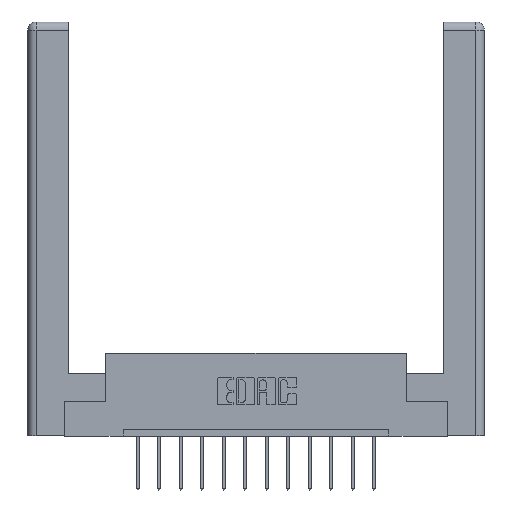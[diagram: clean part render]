
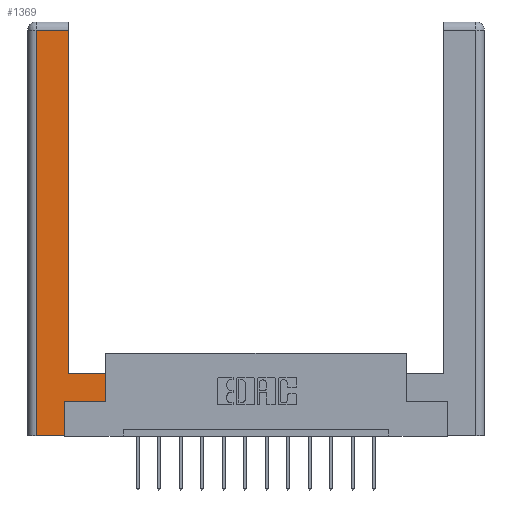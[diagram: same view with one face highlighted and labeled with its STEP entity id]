
A CAD part, top view. The second image highlights one B-rep face of the part: STEP entity #1369.
In plain terms, the highlighted planar face has unit normal (0, 0, 1).
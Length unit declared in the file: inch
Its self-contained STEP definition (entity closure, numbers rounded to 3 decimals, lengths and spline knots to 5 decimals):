
#84 = EDGE_CURVE ( 'NONE', #9626, #12899, #12550, .T. ) ;
#454 = EDGE_CURVE ( 'NONE', #13436, #5802, #12744, .T. ) ;
#967 = CARTESIAN_POINT ( 'NONE',  ( 0.565, 0.245, 0. ) ) ;
#1030 = ORIENTED_EDGE ( 'NONE', *, *, #15448, .T. ) ;
#1088 = CARTESIAN_POINT ( 'NONE',  ( 0.0615, 0., 0. ) ) ;
#1291 = VERTEX_POINT ( 'NONE', #6647 ) ;
#1369 = ADVANCED_FACE ( 'NONE', ( #5963 ), #9973, .F. ) ;
#1589 = LINE ( 'NONE', #15009, #4022 ) ;
#1873 = CARTESIAN_POINT ( 'NONE',  ( 0.265, 0.245, 0. ) ) ;
#1996 = EDGE_CURVE ( 'NONE', #12899, #4036, #5397, .T. ) ;
#2289 = CARTESIAN_POINT ( 'NONE',  ( 0.0615, 2.94, 0. ) ) ;
#2764 = EDGE_CURVE ( 'NONE', #1291, #13004, #11936, .T. ) ;
#2910 = LINE ( 'NONE', #1873, #14109 ) ;
#3070 = ORIENTED_EDGE ( 'NONE', *, *, #1996, .T. ) ;
#3510 = EDGE_LOOP ( 'NONE', ( #1030, #5829, #11685, #3070, #14769, #4694, #4431, #4227 ) ) ;
#3810 = DIRECTION ( 'NONE',  ( 0., 1., 0. ) ) ;
#4022 = VECTOR ( 'NONE', #10203, 39.37008 ) ;
#4036 = VERTEX_POINT ( 'NONE', #5295 ) ;
#4135 = DIRECTION ( 'NONE',  ( 0., 0., -1. ) ) ;
#4186 = CARTESIAN_POINT ( 'NONE',  ( 0., 0., 0. ) ) ;
#4227 = ORIENTED_EDGE ( 'NONE', *, *, #454, .T. ) ;
#4431 = ORIENTED_EDGE ( 'NONE', *, *, #12311, .T. ) ;
#4521 = VECTOR ( 'NONE', #15056, 39.37008 ) ;
#4586 = DIRECTION ( 'NONE',  ( -1., 0., 0. ) ) ;
#4694 = ORIENTED_EDGE ( 'NONE', *, *, #2764, .T. ) ;
#4949 = EDGE_CURVE ( 'NONE', #9069, #9626, #10179, .T. ) ;
#5267 = DIRECTION ( 'NONE',  ( -1., 0., 0. ) ) ;
#5295 = CARTESIAN_POINT ( 'NONE',  ( 0.265, 0., 0. ) ) ;
#5397 = LINE ( 'NONE', #14403, #10457 ) ;
#5498 = CARTESIAN_POINT ( 'NONE',  ( 0.295, 0.45, 0. ) ) ;
#5618 = DIRECTION ( 'NONE',  ( 0., 1., 0. ) ) ;
#5802 = VERTEX_POINT ( 'NONE', #6355 ) ;
#5829 = ORIENTED_EDGE ( 'NONE', *, *, #4949, .T. ) ;
#5963 = FACE_OUTER_BOUND ( 'NONE', #3510, .T. ) ;
#6355 = CARTESIAN_POINT ( 'NONE',  ( 0.295, 0.45, 0. ) ) ;
#6647 = CARTESIAN_POINT ( 'NONE',  ( 0.265, 0.245, 0. ) ) ;
#6973 = DIRECTION ( 'NONE',  ( 1., 0., 0. ) ) ;
#8461 = CARTESIAN_POINT ( 'NONE',  ( 0.295, 2.94, 0. ) ) ;
#8930 = CARTESIAN_POINT ( 'NONE',  ( 0.0615, 0., 0. ) ) ;
#8996 = VECTOR ( 'NONE', #11958, 39.37008 ) ;
#9069 = VERTEX_POINT ( 'NONE', #8461 ) ;
#9594 = VECTOR ( 'NONE', #3810, 39.37008 ) ;
#9626 = VERTEX_POINT ( 'NONE', #14780 ) ;
#9973 = PLANE ( 'NONE',  #10211 ) ;
#9989 = LINE ( 'NONE', #11084, #9594 ) ;
#10179 = LINE ( 'NONE', #2289, #14261 ) ;
#10203 = DIRECTION ( 'NONE',  ( 0., 1., 0. ) ) ;
#10211 = AXIS2_PLACEMENT_3D ( 'NONE', #4186, #4135, #5267 ) ;
#10457 = VECTOR ( 'NONE', #13263, 39.37008 ) ;
#10995 = EDGE_CURVE ( 'NONE', #4036, #1291, #2910, .T. ) ;
#11084 = CARTESIAN_POINT ( 'NONE',  ( 0.295, 3., 0. ) ) ;
#11685 = ORIENTED_EDGE ( 'NONE', *, *, #84, .T. ) ;
#11936 = LINE ( 'NONE', #14202, #15330 ) ;
#11958 = DIRECTION ( 'NONE',  ( 0., -1., 0. ) ) ;
#12311 = EDGE_CURVE ( 'NONE', #13004, #13436, #1589, .T. ) ;
#12550 = LINE ( 'NONE', #1088, #8996 ) ;
#12744 = LINE ( 'NONE', #5498, #4521 ) ;
#12899 = VERTEX_POINT ( 'NONE', #8930 ) ;
#13004 = VERTEX_POINT ( 'NONE', #967 ) ;
#13263 = DIRECTION ( 'NONE',  ( 1., 0., 0. ) ) ;
#13436 = VERTEX_POINT ( 'NONE', #14896 ) ;
#14109 = VECTOR ( 'NONE', #5618, 39.37008 ) ;
#14202 = CARTESIAN_POINT ( 'NONE',  ( 0.565, 0.245, 0. ) ) ;
#14261 = VECTOR ( 'NONE', #4586, 39.37008 ) ;
#14403 = CARTESIAN_POINT ( 'NONE',  ( 0.265, 0., 0. ) ) ;
#14769 = ORIENTED_EDGE ( 'NONE', *, *, #10995, .T. ) ;
#14780 = CARTESIAN_POINT ( 'NONE',  ( 0.0615, 2.94, 0. ) ) ;
#14896 = CARTESIAN_POINT ( 'NONE',  ( 0.565, 0.45, 0. ) ) ;
#15009 = CARTESIAN_POINT ( 'NONE',  ( 0.565, 0.45, 0. ) ) ;
#15056 = DIRECTION ( 'NONE',  ( -1., 0., 0. ) ) ;
#15330 = VECTOR ( 'NONE', #6973, 39.37008 ) ;
#15448 = EDGE_CURVE ( 'NONE', #5802, #9069, #9989, .T. ) ;
